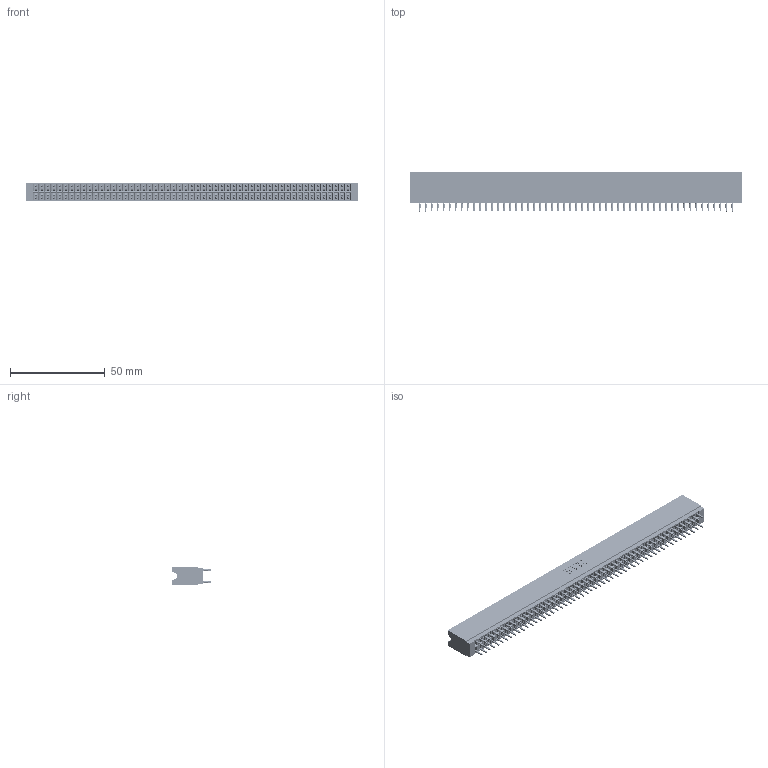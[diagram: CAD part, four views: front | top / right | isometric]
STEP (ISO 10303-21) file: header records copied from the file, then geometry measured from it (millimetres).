
FILE_DESCRIPTION (( 'STEP AP203' ), '1' );
FILE_NAME ('746-106-560-206.STEP', '2026-03-04T23:57:02', ( '' ), ( '' ), 'SwSTEP 2.0', 'SolidWorks 2023', '' );
FILE_SCHEMA (( 'CONFIG_CONTROL_DESIGN' ));
Length unit declared in the file: millimetre
Products named in the file (3): 746 Part_.515 Slot Depth - 06; 746-292-001_560; 746-106-560-206
Assembly tree (107 placements, depth 2):
  746-106-560-206
    746 Part_.515 Slot Depth - 06
    746-292-001_560  x106
Bounding box: 175.51 x 20.82 x 9.91 mm (x, y, z)
Volume: 19086.7 mm3; surface area: 32615.6 mm2
Topology: 107 solids, 107 shells, 10115 faces, 28143 edges, 18036 vertices
Faces by surface type: plane 5038, cylinder 2321, bspline 2120, torus 636
Entity records: 80442 total; most frequent: CARTESIAN_POINT 15892, ORIENTED_EDGE 13866, DIRECTION 11565, EDGE_CURVE 6933, LINE 6211, VECTOR 6211, VERTEX_POINT 4596, AXIS2_PLACEMENT_3D 2677
